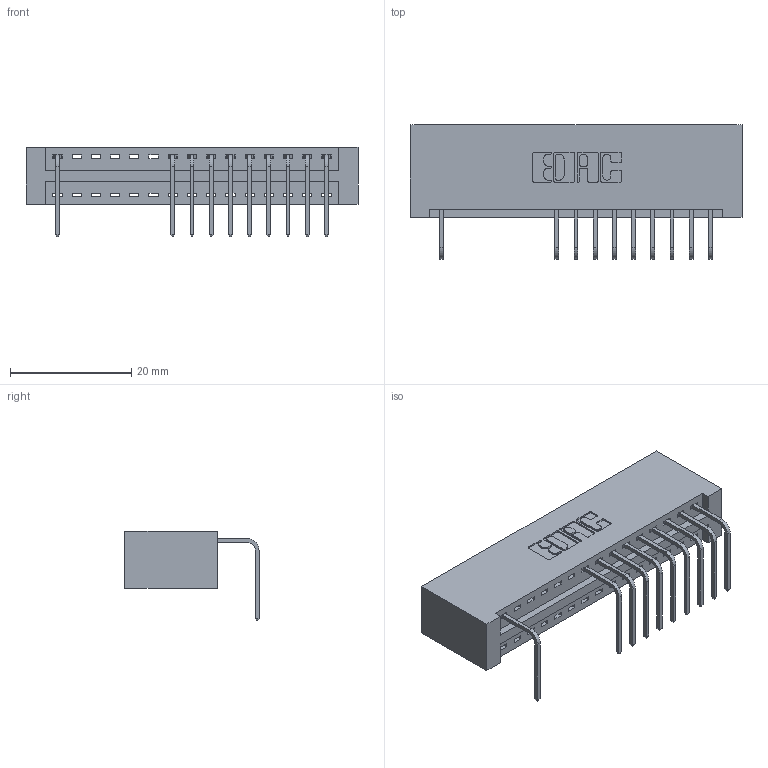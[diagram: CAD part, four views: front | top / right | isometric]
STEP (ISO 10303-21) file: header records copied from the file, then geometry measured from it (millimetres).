
FILE_DESCRIPTION (( 'STEP AP203' ), '1' );
FILE_NAME ('346-015-558-101.STEP', '2018-08-20T03:03:34', ( '' ), ( '' ), 'SwSTEP 2.0', 'SolidWorks 2016', '' );
FILE_SCHEMA (( 'CONFIG_CONTROL_DESIGN' ));
Length unit declared in the file: inch
Products named in the file (3): 345-292-001_558 Tail - 2; 346-015-558-101; 346 Part_No Mounting Lugs
Assembly tree (11 placements, depth 2):
  346-015-558-101
    346 Part_No Mounting Lugs
    345-292-001_558 Tail - 2  x10
Bounding box: 54.86 x 22.16 x 14.73 mm (x, y, z)
Volume: 5591.2 mm3; surface area: 6663.1 mm2
Topology: 11 solids, 11 shells, 774 faces, 2335 edges, 1542 vertices
Faces by surface type: plane 542, cylinder 232
Entity records: 12591 total; most frequent: CARTESIAN_POINT 2196, ORIENTED_EDGE 2150, DIRECTION 1959, EDGE_CURVE 1075, VECTOR 891, LINE 891, VERTEX_POINT 714, AXIS2_PLACEMENT_3D 534
